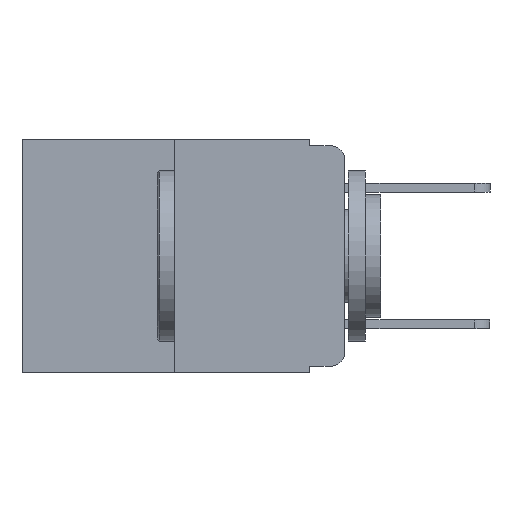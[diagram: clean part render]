
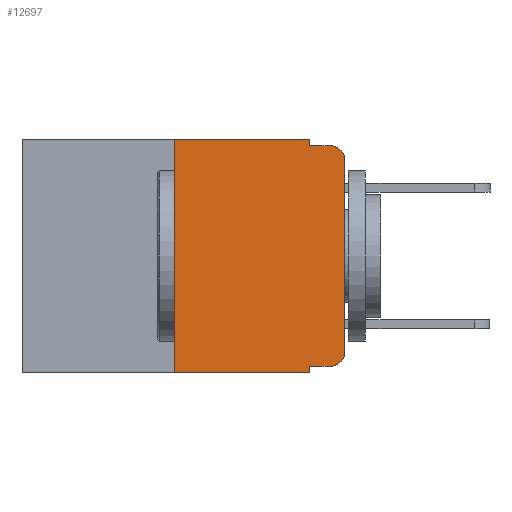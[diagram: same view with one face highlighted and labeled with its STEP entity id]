
A CAD part, left-side view. The second image highlights one B-rep face of the part: STEP entity #12697.
In plain terms, the highlighted planar face has unit normal (-1, 0, 0).
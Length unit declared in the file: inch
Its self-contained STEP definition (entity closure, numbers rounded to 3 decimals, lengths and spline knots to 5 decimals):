
#34 = VERTEX_POINT ( 'NONE', #14154 ) ;
#149 = DIRECTION ( 'NONE',  ( 0., -1., 0. ) ) ;
#181 = CARTESIAN_POINT ( 'NONE',  ( 0., 0., -0.313 ) ) ;
#311 = CARTESIAN_POINT ( 'NONE',  ( 0., 0.051, -0.01 ) ) ;
#429 = ORIENTED_EDGE ( 'NONE', *, *, #18165, .T. ) ;
#514 = DIRECTION ( 'NONE',  ( 0., 0., -1. ) ) ;
#706 = VERTEX_POINT ( 'NONE', #3114 ) ;
#900 = VECTOR ( 'NONE', #12871, 39.37008 ) ;
#985 = CARTESIAN_POINT ( 'NONE',  ( 0., 0.473, -0.343 ) ) ;
#1153 = EDGE_LOOP ( 'NONE', ( #7044, #6799, #8852, #8321, #7847, #5512, #429, #3117, #18185, #2138 ) ) ;
#1291 = CARTESIAN_POINT ( 'NONE',  ( 0., 0.02, -0.03 ) ) ;
#1744 = VERTEX_POINT ( 'NONE', #17776 ) ;
#2138 = ORIENTED_EDGE ( 'NONE', *, *, #11218, .T. ) ;
#2383 = VERTEX_POINT ( 'NONE', #181 ) ;
#2435 = VERTEX_POINT ( 'NONE', #311 ) ;
#2631 = LINE ( 'NONE', #8444, #14498 ) ;
#2862 = CIRCLE ( 'NONE', #3414, 0.02 ) ;
#3009 = DIRECTION ( 'NONE',  ( 0., 0., -1. ) ) ;
#3114 = CARTESIAN_POINT ( 'NONE',  ( 0., 0.051, -0.343 ) ) ;
#3117 = ORIENTED_EDGE ( 'NONE', *, *, #17708, .F. ) ;
#3303 = EDGE_CURVE ( 'NONE', #1744, #2435, #9875, .T. ) ;
#3414 = AXIS2_PLACEMENT_3D ( 'NONE', #18678, #10374, #514 ) ;
#3966 = CARTESIAN_POINT ( 'NONE',  ( 0., 0.051, 0. ) ) ;
#4012 = CARTESIAN_POINT ( 'NONE',  ( 0., 0., 0. ) ) ;
#4462 = EDGE_CURVE ( 'NONE', #2435, #5683, #2631, .T. ) ;
#4577 = VECTOR ( 'NONE', #19035, 39.37008 ) ;
#4754 = DIRECTION ( 'NONE',  ( 0., 0., -1. ) ) ;
#5512 = ORIENTED_EDGE ( 'NONE', *, *, #19501, .F. ) ;
#5526 = VERTEX_POINT ( 'NONE', #9973 ) ;
#5683 = VERTEX_POINT ( 'NONE', #8749 ) ;
#6147 = VECTOR ( 'NONE', #4754, 39.37008 ) ;
#6237 = LINE ( 'NONE', #4012, #17823 ) ;
#6706 = EDGE_CURVE ( 'NONE', #12589, #5683, #14225, .T. ) ;
#6799 = ORIENTED_EDGE ( 'NONE', *, *, #6706, .T. ) ;
#7044 = ORIENTED_EDGE ( 'NONE', *, *, #7754, .T. ) ;
#7098 = CARTESIAN_POINT ( 'NONE',  ( 0., 0.25, 0. ) ) ;
#7754 = EDGE_CURVE ( 'NONE', #2383, #12589, #6237, .T. ) ;
#7847 = ORIENTED_EDGE ( 'NONE', *, *, #13626, .F. ) ;
#8224 = FACE_OUTER_BOUND ( 'NONE', #1153, .T. ) ;
#8321 = ORIENTED_EDGE ( 'NONE', *, *, #3303, .F. ) ;
#8444 = CARTESIAN_POINT ( 'NONE',  ( 0., 0.051, -0.01 ) ) ;
#8749 = CARTESIAN_POINT ( 'NONE',  ( 0., 0.02, -0.01 ) ) ;
#8852 = ORIENTED_EDGE ( 'NONE', *, *, #4462, .F. ) ;
#8893 = DIRECTION ( 'NONE',  ( 0., 0., 1. ) ) ;
#8898 = LINE ( 'NONE', #985, #4577 ) ;
#8929 = CARTESIAN_POINT ( 'NONE',  ( 0., 0.473, 0. ) ) ;
#9139 = VERTEX_POINT ( 'NONE', #7098 ) ;
#9284 = DIRECTION ( 'NONE',  ( 1., 0., 0. ) ) ;
#9875 = LINE ( 'NONE', #3966, #16468 ) ;
#9973 = CARTESIAN_POINT ( 'NONE',  ( 0., 0.25, -0.343 ) ) ;
#10374 = DIRECTION ( 'NONE',  ( -1., 0., 0. ) ) ;
#10384 = DIRECTION ( 'NONE',  ( 0., 0., -1. ) ) ;
#10426 = AXIS2_PLACEMENT_3D ( 'NONE', #1291, #12462, #3009 ) ;
#10859 = AXIS2_PLACEMENT_3D ( 'NONE', #8929, #9284, #19054 ) ;
#11175 = VECTOR ( 'NONE', #14029, 39.37008 ) ;
#11218 = EDGE_CURVE ( 'NONE', #17245, #2383, #2862, .T. ) ;
#11445 = CARTESIAN_POINT ( 'NONE',  ( 0., 0.051, -0.333 ) ) ;
#11498 = CARTESIAN_POINT ( 'NONE',  ( 0., 0.02, -0.333 ) ) ;
#11617 = LINE ( 'NONE', #15409, #11175 ) ;
#12462 = DIRECTION ( 'NONE',  ( -1., 0., 0. ) ) ;
#12589 = VERTEX_POINT ( 'NONE', #18515 ) ;
#12617 = VECTOR ( 'NONE', #16576, 39.37008 ) ;
#12697 = ADVANCED_FACE ( 'NONE', ( #8224 ), #16318, .F. ) ;
#12871 = DIRECTION ( 'NONE',  ( 0., -1., 0. ) ) ;
#13069 = LINE ( 'NONE', #15219, #12617 ) ;
#13117 = EDGE_CURVE ( 'NONE', #34, #17245, #17580, .T. ) ;
#13626 = EDGE_CURVE ( 'NONE', #9139, #1744, #13069, .T. ) ;
#14029 = DIRECTION ( 'NONE',  ( 0., 0., 1. ) ) ;
#14116 = LINE ( 'NONE', #15269, #6147 ) ;
#14154 = CARTESIAN_POINT ( 'NONE',  ( 0., 0.051, -0.333 ) ) ;
#14225 = CIRCLE ( 'NONE', #10426, 0.02 ) ;
#14498 = VECTOR ( 'NONE', #149, 39.37008 ) ;
#15219 = CARTESIAN_POINT ( 'NONE',  ( 0., 0.473, 0. ) ) ;
#15269 = CARTESIAN_POINT ( 'NONE',  ( 0., 0.051, 0. ) ) ;
#15409 = CARTESIAN_POINT ( 'NONE',  ( 0., 0.25, 0. ) ) ;
#16318 = PLANE ( 'NONE',  #10859 ) ;
#16468 = VECTOR ( 'NONE', #10384, 39.37008 ) ;
#16576 = DIRECTION ( 'NONE',  ( 0., -1., 0. ) ) ;
#17245 = VERTEX_POINT ( 'NONE', #11498 ) ;
#17580 = LINE ( 'NONE', #11445, #900 ) ;
#17708 = EDGE_CURVE ( 'NONE', #34, #706, #14116, .T. ) ;
#17776 = CARTESIAN_POINT ( 'NONE',  ( 0., 0.051, 0. ) ) ;
#17823 = VECTOR ( 'NONE', #8893, 39.37008 ) ;
#18165 = EDGE_CURVE ( 'NONE', #5526, #706, #8898, .T. ) ;
#18185 = ORIENTED_EDGE ( 'NONE', *, *, #13117, .T. ) ;
#18515 = CARTESIAN_POINT ( 'NONE',  ( 0., 0., -0.03 ) ) ;
#18678 = CARTESIAN_POINT ( 'NONE',  ( 0., 0.02, -0.313 ) ) ;
#19035 = DIRECTION ( 'NONE',  ( 0., -1., 0. ) ) ;
#19054 = DIRECTION ( 'NONE',  ( 0., 0., -1. ) ) ;
#19501 = EDGE_CURVE ( 'NONE', #5526, #9139, #11617, .T. ) ;
